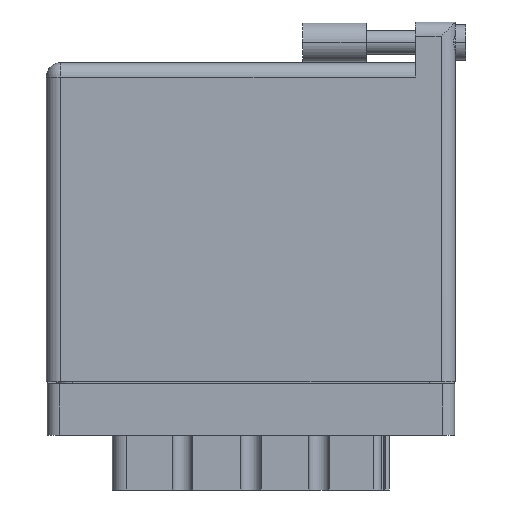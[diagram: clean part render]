
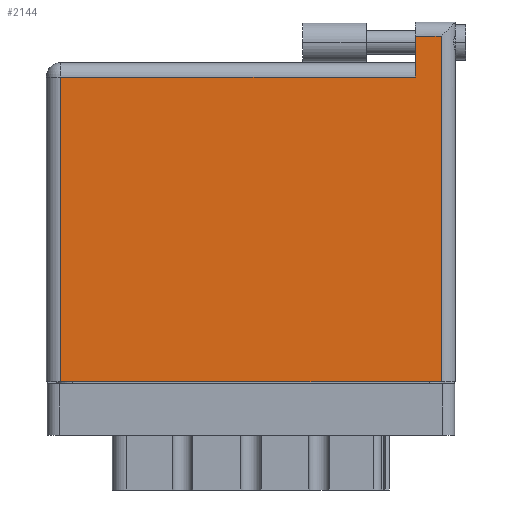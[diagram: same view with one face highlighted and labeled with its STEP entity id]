
A CAD part, front view. The second image highlights one B-rep face of the part: STEP entity #2144.
In plain terms, the highlighted face is planar.
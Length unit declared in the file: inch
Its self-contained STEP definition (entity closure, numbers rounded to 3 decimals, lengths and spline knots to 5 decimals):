
#315 = VERTEX_POINT ( 'NONE', #17068 ) ;
#526 = ORIENTED_EDGE ( 'NONE', *, *, #32330, .T. ) ;
#1144 = LINE ( 'NONE', #32760, #30562 ) ;
#1352 = CARTESIAN_POINT ( 'NONE',  ( 1.811, 1.696, 0. ) ) ;
#2144 = ADVANCED_FACE ( 'NONE', ( #31758 ), #33786, .F. ) ;
#3824 = LINE ( 'NONE', #22024, #23479 ) ;
#3942 = ORIENTED_EDGE ( 'NONE', *, *, #26149, .T. ) ;
#4363 = LINE ( 'NONE', #33530, #15079 ) ;
#4565 = DIRECTION ( 'NONE',  ( 1., 0., 0. ) ) ;
#4749 = ORIENTED_EDGE ( 'NONE', *, *, #21741, .T. ) ;
#5460 = LINE ( 'NONE', #36051, #7261 ) ;
#6857 = CARTESIAN_POINT ( 'NONE',  ( 1.938, 1.766, 0. ) ) ;
#7261 = VECTOR ( 'NONE', #13853, 39.37008 ) ;
#7793 = VERTEX_POINT ( 'NONE', #1352 ) ;
#8335 = DIRECTION ( 'NONE',  ( 0., -1., 0. ) ) ;
#8442 = ORIENTED_EDGE ( 'NONE', *, *, #11975, .T. ) ;
#8931 = EDGE_CURVE ( 'NONE', #7793, #14510, #4363, .T. ) ;
#10451 = DIRECTION ( 'NONE',  ( -1., 0., 0. ) ) ;
#10543 = EDGE_LOOP ( 'NONE', ( #11330, #4749, #526, #34480, #8442, #3942 ) ) ;
#11330 = ORIENTED_EDGE ( 'NONE', *, *, #14675, .T. ) ;
#11975 = EDGE_CURVE ( 'NONE', #14510, #315, #5460, .T. ) ;
#13780 = VERTEX_POINT ( 'NONE', #32315 ) ;
#13853 = DIRECTION ( 'NONE',  ( -1., 0., 0. ) ) ;
#13876 = LINE ( 'NONE', #6857, #29957 ) ;
#14510 = VERTEX_POINT ( 'NONE', #18272 ) ;
#14675 = EDGE_CURVE ( 'NONE', #25290, #13780, #1144, .T. ) ;
#14825 = VERTEX_POINT ( 'NONE', #22275 ) ;
#15079 = VECTOR ( 'NONE', #8335, 39.37008 ) ;
#16674 = DIRECTION ( 'NONE',  ( 0., 0., -1. ) ) ;
#17068 = CARTESIAN_POINT ( 'NONE',  ( 0.07, 1.496, 0. ) ) ;
#17965 = LINE ( 'NONE', #25994, #28232 ) ;
#18272 = CARTESIAN_POINT ( 'NONE',  ( 1.811, 1.496, 0. ) ) ;
#19667 = CARTESIAN_POINT ( 'NONE',  ( 0.07, 0., 0. ) ) ;
#21741 = EDGE_CURVE ( 'NONE', #13780, #14825, #13876, .T. ) ;
#22024 = CARTESIAN_POINT ( 'NONE',  ( 0., 1.696, 0. ) ) ;
#22275 = CARTESIAN_POINT ( 'NONE',  ( 1.938, 1.696, 0. ) ) ;
#23479 = VECTOR ( 'NONE', #28117, 39.37008 ) ;
#23500 = DIRECTION ( 'NONE',  ( 0., -1., 0. ) ) ;
#25290 = VERTEX_POINT ( 'NONE', #19667 ) ;
#25994 = CARTESIAN_POINT ( 'NONE',  ( 0.07, 0., 0. ) ) ;
#26149 = EDGE_CURVE ( 'NONE', #315, #25290, #17965, .T. ) ;
#26468 = AXIS2_PLACEMENT_3D ( 'NONE', #36132, #16674, #10451 ) ;
#26816 = DIRECTION ( 'NONE',  ( 0., 1., 0. ) ) ;
#28117 = DIRECTION ( 'NONE',  ( -1., 0., 0. ) ) ;
#28232 = VECTOR ( 'NONE', #23500, 39.37008 ) ;
#29957 = VECTOR ( 'NONE', #26816, 39.37008 ) ;
#30562 = VECTOR ( 'NONE', #4565, 39.37008 ) ;
#31758 = FACE_OUTER_BOUND ( 'NONE', #10543, .T. ) ;
#32315 = CARTESIAN_POINT ( 'NONE',  ( 1.938, 0., 0. ) ) ;
#32330 = EDGE_CURVE ( 'NONE', #14825, #7793, #3824, .T. ) ;
#32760 = CARTESIAN_POINT ( 'NONE',  ( 0., 0., 0. ) ) ;
#33530 = CARTESIAN_POINT ( 'NONE',  ( 1.811, 1.766, 0. ) ) ;
#33786 = PLANE ( 'NONE',  #26468 ) ;
#34480 = ORIENTED_EDGE ( 'NONE', *, *, #8931, .T. ) ;
#36051 = CARTESIAN_POINT ( 'NONE',  ( 0., 1.496, 0. ) ) ;
#36132 = CARTESIAN_POINT ( 'NONE',  ( 0., 1.566, 0. ) ) ;
